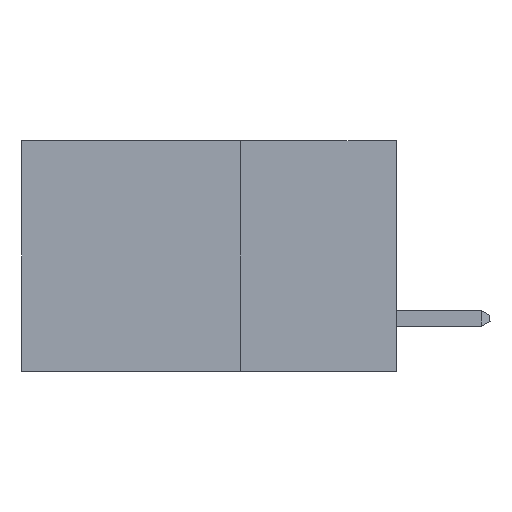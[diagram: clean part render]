
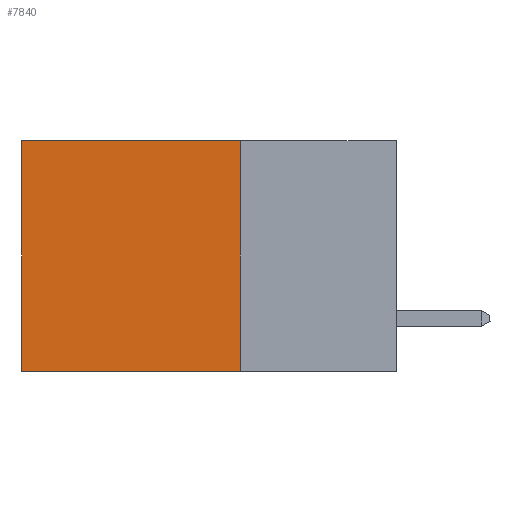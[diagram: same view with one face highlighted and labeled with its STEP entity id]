
A CAD part, left-side view. The second image highlights one B-rep face of the part: STEP entity #7840.
In plain terms, the highlighted planar face has unit normal (-1, 0, 0).
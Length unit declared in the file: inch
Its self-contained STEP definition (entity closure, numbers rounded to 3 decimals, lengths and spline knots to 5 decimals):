
#432 = LINE ( 'NONE', #8127, #3653 ) ;
#555 = DIRECTION ( 'NONE',  ( 0., 1., 0. ) ) ;
#1257 = DIRECTION ( 'NONE',  ( 0., 0., -1. ) ) ;
#1417 = DIRECTION ( 'NONE',  ( 0., 0., -1. ) ) ;
#1535 = VECTOR ( 'NONE', #12082, 39.37008 ) ;
#1748 = ORIENTED_EDGE ( 'NONE', *, *, #13419, .F. ) ;
#2138 = CARTESIAN_POINT ( 'NONE',  ( 0.298, 0.6, -0.37 ) ) ;
#3046 = ORIENTED_EDGE ( 'NONE', *, *, #7174, .F. ) ;
#3653 = VECTOR ( 'NONE', #1257, 39.37008 ) ;
#4830 = ORIENTED_EDGE ( 'NONE', *, *, #5306, .T. ) ;
#5306 = EDGE_CURVE ( 'NONE', #9667, #8364, #17304, .T. ) ;
#5932 = CARTESIAN_POINT ( 'NONE',  ( 0.298, 0.25, 0. ) ) ;
#6644 = CARTESIAN_POINT ( 'NONE',  ( 0.298, 0.25, 0. ) ) ;
#6751 = DIRECTION ( 'NONE',  ( 1., 0., 0. ) ) ;
#6803 = CARTESIAN_POINT ( 'NONE',  ( 0.298, 0.25, 0. ) ) ;
#7174 = EDGE_CURVE ( 'NONE', #9667, #14529, #17013, .T. ) ;
#7285 = CARTESIAN_POINT ( 'NONE',  ( 0.298, 0.25, 0. ) ) ;
#7840 = ADVANCED_FACE ( 'NONE', ( #10821 ), #9181, .F. ) ;
#8127 = CARTESIAN_POINT ( 'NONE',  ( 0.298, 0.6, 0. ) ) ;
#8364 = VERTEX_POINT ( 'NONE', #14282 ) ;
#8790 = VECTOR ( 'NONE', #555, 39.37008 ) ;
#9181 = PLANE ( 'NONE',  #9320 ) ;
#9320 = AXIS2_PLACEMENT_3D ( 'NONE', #6644, #6751, #16380 ) ;
#9667 = VERTEX_POINT ( 'NONE', #5932 ) ;
#10821 = FACE_OUTER_BOUND ( 'NONE', #15565, .T. ) ;
#12082 = DIRECTION ( 'NONE',  ( 0., 1., 0. ) ) ;
#12205 = LINE ( 'NONE', #13658, #1535 ) ;
#12943 = CARTESIAN_POINT ( 'NONE',  ( 0.298, 0.25, -0.37 ) ) ;
#13419 = EDGE_CURVE ( 'NONE', #14529, #15080, #12205, .T. ) ;
#13658 = CARTESIAN_POINT ( 'NONE',  ( 0.298, 0.25, -0.37 ) ) ;
#13739 = EDGE_CURVE ( 'NONE', #8364, #15080, #432, .T. ) ;
#14282 = CARTESIAN_POINT ( 'NONE',  ( 0.298, 0.6, 0. ) ) ;
#14529 = VERTEX_POINT ( 'NONE', #12943 ) ;
#14874 = VECTOR ( 'NONE', #1417, 39.37008 ) ;
#15080 = VERTEX_POINT ( 'NONE', #2138 ) ;
#15565 = EDGE_LOOP ( 'NONE', ( #15623, #1748, #3046, #4830 ) ) ;
#15623 = ORIENTED_EDGE ( 'NONE', *, *, #13739, .T. ) ;
#16380 = DIRECTION ( 'NONE',  ( 0., 0., -1. ) ) ;
#17013 = LINE ( 'NONE', #6803, #14874 ) ;
#17304 = LINE ( 'NONE', #7285, #8790 ) ;
